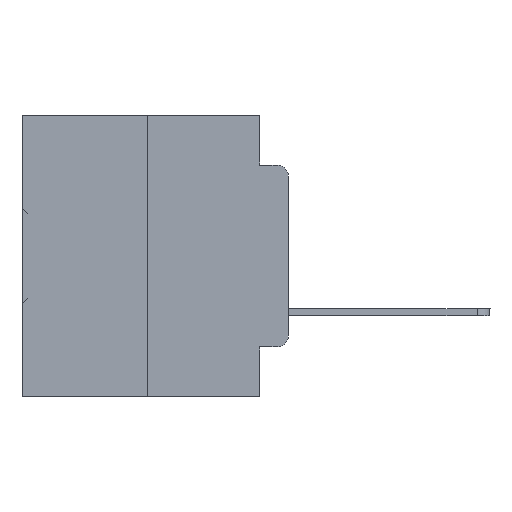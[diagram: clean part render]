
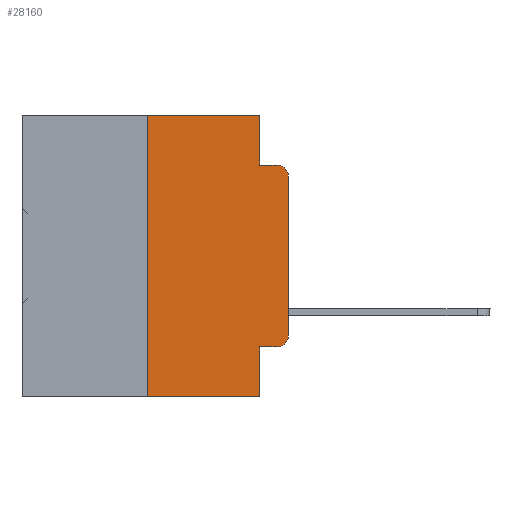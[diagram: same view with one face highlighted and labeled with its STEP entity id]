
A CAD part, left-side view. The second image highlights one B-rep face of the part: STEP entity #28160.
In plain terms, the highlighted planar face has unit normal (-1, 0, 0).
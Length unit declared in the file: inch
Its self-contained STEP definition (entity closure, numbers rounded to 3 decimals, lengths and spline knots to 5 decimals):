
#293 = CARTESIAN_POINT ( 'NONE',  ( 0., 0.473, 0. ) ) ;
#1155 = ORIENTED_EDGE ( 'NONE', *, *, #32255, .T. ) ;
#1398 = CARTESIAN_POINT ( 'NONE',  ( 0., 0.051, -0.5 ) ) ;
#1941 = DIRECTION ( 'NONE',  ( 0., 0., -1. ) ) ;
#1997 = EDGE_CURVE ( 'NONE', #34410, #36042, #15903, .T. ) ;
#2032 = VECTOR ( 'NONE', #19217, 39.37008 ) ;
#2166 = DIRECTION ( 'NONE',  ( 0., -1., 0. ) ) ;
#2214 = ORIENTED_EDGE ( 'NONE', *, *, #5488, .F. ) ;
#2559 = ORIENTED_EDGE ( 'NONE', *, *, #1997, .T. ) ;
#3406 = EDGE_CURVE ( 'NONE', #36042, #8904, #34206, .T. ) ;
#3533 = AXIS2_PLACEMENT_3D ( 'NONE', #21164, #24034, #35592 ) ;
#4148 = VERTEX_POINT ( 'NONE', #13960 ) ;
#4387 = CARTESIAN_POINT ( 'NONE',  ( 0., 0., 0. ) ) ;
#4891 = CARTESIAN_POINT ( 'NONE',  ( 0., 0.473, 0. ) ) ;
#5228 = VERTEX_POINT ( 'NONE', #13893 ) ;
#5309 = VERTEX_POINT ( 'NONE', #34949 ) ;
#5439 = CARTESIAN_POINT ( 'NONE',  ( 0., 0.02, -0.3915 ) ) ;
#5488 = EDGE_CURVE ( 'NONE', #5309, #28342, #19112, .T. ) ;
#6409 = ORIENTED_EDGE ( 'NONE', *, *, #13160, .T. ) ;
#6823 = DIRECTION ( 'NONE',  ( 0., 0., -1. ) ) ;
#7344 = AXIS2_PLACEMENT_3D ( 'NONE', #293, #11909, #12154 ) ;
#8241 = CARTESIAN_POINT ( 'NONE',  ( 0., 0.051, -0.4115 ) ) ;
#8904 = VERTEX_POINT ( 'NONE', #27238 ) ;
#9909 = LINE ( 'NONE', #36397, #17110 ) ;
#10272 = VERTEX_POINT ( 'NONE', #8241 ) ;
#10274 = AXIS2_PLACEMENT_3D ( 'NONE', #5439, #27890, #36931 ) ;
#11327 = CARTESIAN_POINT ( 'NONE',  ( 0., 0.473, -0.5 ) ) ;
#11592 = VERTEX_POINT ( 'NONE', #17799 ) ;
#11716 = VERTEX_POINT ( 'NONE', #1398 ) ;
#11775 = VECTOR ( 'NONE', #6823, 39.37008 ) ;
#11909 = DIRECTION ( 'NONE',  ( 1., 0., 0. ) ) ;
#12154 = DIRECTION ( 'NONE',  ( 0., 0., -1. ) ) ;
#13160 = EDGE_CURVE ( 'NONE', #8904, #5228, #18580, .T. ) ;
#13531 = DIRECTION ( 'NONE',  ( 0., -1., 0. ) ) ;
#13893 = CARTESIAN_POINT ( 'NONE',  ( 0., 0.02, -0.0885 ) ) ;
#13960 = CARTESIAN_POINT ( 'NONE',  ( 0., 0.051, -0.0885 ) ) ;
#14028 = VECTOR ( 'NONE', #24448, 39.37008 ) ;
#14453 = VECTOR ( 'NONE', #23651, 39.37008 ) ;
#15063 = CARTESIAN_POINT ( 'NONE',  ( 0., 0.051, 0. ) ) ;
#15345 = ORIENTED_EDGE ( 'NONE', *, *, #31099, .F. ) ;
#15450 = LINE ( 'NONE', #19714, #2032 ) ;
#15903 = CIRCLE ( 'NONE', #10274, 0.02 ) ;
#16163 = ORIENTED_EDGE ( 'NONE', *, *, #28586, .F. ) ;
#16620 = LINE ( 'NONE', #11327, #29566 ) ;
#16702 = LINE ( 'NONE', #33404, #36902 ) ;
#17110 = VECTOR ( 'NONE', #2166, 39.37008 ) ;
#17721 = VECTOR ( 'NONE', #13531, 39.37008 ) ;
#17799 = CARTESIAN_POINT ( 'NONE',  ( 0., 0.25, -0.5 ) ) ;
#18083 = CARTESIAN_POINT ( 'NONE',  ( 0., 0.051, 0. ) ) ;
#18376 = EDGE_CURVE ( 'NONE', #10272, #11716, #16702, .T. ) ;
#18580 = CIRCLE ( 'NONE', #3533, 0.02 ) ;
#19112 = LINE ( 'NONE', #4891, #17721 ) ;
#19217 = DIRECTION ( 'NONE',  ( 0., 0., 1. ) ) ;
#19714 = CARTESIAN_POINT ( 'NONE',  ( 0., 0.25, 0. ) ) ;
#20168 = ORIENTED_EDGE ( 'NONE', *, *, #31473, .T. ) ;
#21164 = CARTESIAN_POINT ( 'NONE',  ( 0., 0.02, -0.1085 ) ) ;
#23651 = DIRECTION ( 'NONE',  ( 0., -1., 0. ) ) ;
#24034 = DIRECTION ( 'NONE',  ( -1., 0., 0. ) ) ;
#24448 = DIRECTION ( 'NONE',  ( 0., 0., 1. ) ) ;
#25812 = FACE_OUTER_BOUND ( 'NONE', #36755, .T. ) ;
#26067 = DIRECTION ( 'NONE',  ( 0., -1., 0. ) ) ;
#26122 = ORIENTED_EDGE ( 'NONE', *, *, #3406, .T. ) ;
#26440 = PLANE ( 'NONE',  #7344 ) ;
#27238 = CARTESIAN_POINT ( 'NONE',  ( 0., 0., -0.1085 ) ) ;
#27890 = DIRECTION ( 'NONE',  ( -1., 0., 0. ) ) ;
#28160 = ADVANCED_FACE ( 'NONE', ( #25812 ), #26440, .F. ) ;
#28342 = VERTEX_POINT ( 'NONE', #15063 ) ;
#28586 = EDGE_CURVE ( 'NONE', #11592, #5309, #15450, .T. ) ;
#29210 = LINE ( 'NONE', #34610, #14453 ) ;
#29566 = VECTOR ( 'NONE', #26067, 39.37008 ) ;
#30157 = ORIENTED_EDGE ( 'NONE', *, *, #30645, .F. ) ;
#30645 = EDGE_CURVE ( 'NONE', #28342, #4148, #34679, .T. ) ;
#31099 = EDGE_CURVE ( 'NONE', #4148, #5228, #29210, .T. ) ;
#31473 = EDGE_CURVE ( 'NONE', #10272, #34410, #9909, .T. ) ;
#32232 = ORIENTED_EDGE ( 'NONE', *, *, #18376, .F. ) ;
#32255 = EDGE_CURVE ( 'NONE', #11592, #11716, #16620, .T. ) ;
#33404 = CARTESIAN_POINT ( 'NONE',  ( 0., 0.051, 0. ) ) ;
#33496 = CARTESIAN_POINT ( 'NONE',  ( 0., 0.02, -0.4115 ) ) ;
#34206 = LINE ( 'NONE', #4387, #14028 ) ;
#34410 = VERTEX_POINT ( 'NONE', #33496 ) ;
#34610 = CARTESIAN_POINT ( 'NONE',  ( 0., 0.051, -0.0885 ) ) ;
#34679 = LINE ( 'NONE', #18083, #11775 ) ;
#34949 = CARTESIAN_POINT ( 'NONE',  ( 0., 0.25, 0. ) ) ;
#35215 = CARTESIAN_POINT ( 'NONE',  ( 0., 0., -0.3915 ) ) ;
#35592 = DIRECTION ( 'NONE',  ( 0., 0., -1. ) ) ;
#36042 = VERTEX_POINT ( 'NONE', #35215 ) ;
#36397 = CARTESIAN_POINT ( 'NONE',  ( 0., 0.051, -0.4115 ) ) ;
#36755 = EDGE_LOOP ( 'NONE', ( #26122, #6409, #15345, #30157, #2214, #16163, #1155, #32232, #20168, #2559 ) ) ;
#36902 = VECTOR ( 'NONE', #1941, 39.37008 ) ;
#36931 = DIRECTION ( 'NONE',  ( 0., 0., -1. ) ) ;
